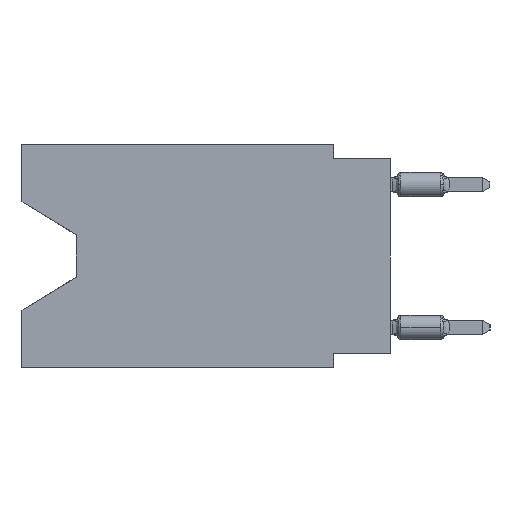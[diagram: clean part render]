
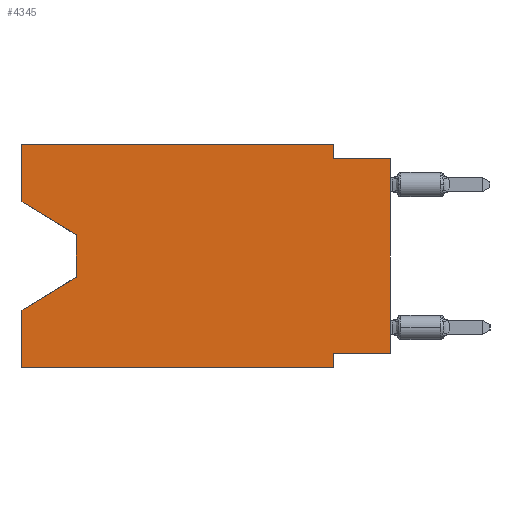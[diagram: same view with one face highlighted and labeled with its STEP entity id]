
A CAD part, left-side view. The second image highlights one B-rep face of the part: STEP entity #4345.
In plain terms, the highlighted planar face has unit normal (-1, 0, 0).
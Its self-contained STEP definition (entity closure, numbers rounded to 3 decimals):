
#278 = ORIENTED_EDGE ( 'NONE', *, *, #27530, .F. ) ;
#301 = LINE ( 'NONE', #47428, #45025 ) ;
#557 = PLANE ( 'NONE',  #7163 ) ;
#610 = DIRECTION ( 'NONE',  ( 0., -1., 0. ) ) ;
#781 = CARTESIAN_POINT ( 'NONE',  ( 0., 16.383, 0. ) ) ;
#833 = FACE_OUTER_BOUND ( 'NONE', #54676, .T. ) ;
#1397 = ORIENTED_EDGE ( 'NONE', *, *, #30987, .F. ) ;
#1782 = DIRECTION ( 'NONE',  ( 0., 0., -1. ) ) ;
#1792 = DIRECTION ( 'NONE',  ( 0., -1., 0. ) ) ;
#1962 = ORIENTED_EDGE ( 'NONE', *, *, #17357, .T. ) ;
#2312 = ORIENTED_EDGE ( 'NONE', *, *, #31524, .T. ) ;
#2405 = DIRECTION ( 'NONE',  ( 0., -1., 0. ) ) ;
#2544 = LINE ( 'NONE', #53923, #33160 ) ;
#3233 = CARTESIAN_POINT ( 'NONE',  ( 0., 2.54, -0.635 ) ) ;
#3855 = ORIENTED_EDGE ( 'NONE', *, *, #21883, .T. ) ;
#4100 = CARTESIAN_POINT ( 'NONE',  ( 0., 13.97, -5.893 ) ) ;
#4287 = LINE ( 'NONE', #25997, #41731 ) ;
#4345 = ADVANCED_FACE ( 'NONE', ( #833 ), #557, .F. ) ;
#5306 = ORIENTED_EDGE ( 'NONE', *, *, #22616, .T. ) ;
#5892 = VERTEX_POINT ( 'NONE', #55152 ) ;
#5977 = CARTESIAN_POINT ( 'NONE',  ( 0., 13.97, -4.013 ) ) ;
#6308 = LINE ( 'NONE', #40852, #37037 ) ;
#7163 = AXIS2_PLACEMENT_3D ( 'NONE', #44235, #23108, #9968 ) ;
#7332 = DIRECTION ( 'NONE',  ( 0., 0., -1. ) ) ;
#8209 = VERTEX_POINT ( 'NONE', #47959 ) ;
#9968 = DIRECTION ( 'NONE',  ( 0., 0., -1. ) ) ;
#11978 = DIRECTION ( 'NONE',  ( 0., -0.855, -0.519 ) ) ;
#12118 = EDGE_CURVE ( 'NONE', #30100, #5892, #39428, .T. ) ;
#13028 = LINE ( 'NONE', #52124, #28872 ) ;
#13922 = VECTOR ( 'NONE', #31520, 1000. ) ;
#14980 = CARTESIAN_POINT ( 'NONE',  ( 0., 0., -0.635 ) ) ;
#15195 = LINE ( 'NONE', #40882, #54041 ) ;
#15851 = EDGE_CURVE ( 'NONE', #8209, #45009, #21567, .T. ) ;
#16890 = DIRECTION ( 'NONE',  ( 0., 1., 0. ) ) ;
#16923 = EDGE_CURVE ( 'NONE', #54320, #50392, #301, .T. ) ;
#17357 = EDGE_CURVE ( 'NONE', #19999, #39767, #34508, .T. ) ;
#17637 = CARTESIAN_POINT ( 'NONE',  ( 0., 16.383, -2.546 ) ) ;
#18548 = VECTOR ( 'NONE', #610, 1000. ) ;
#18921 = CARTESIAN_POINT ( 'NONE',  ( 0., 0., -0.635 ) ) ;
#19999 = VERTEX_POINT ( 'NONE', #55900 ) ;
#20758 = VECTOR ( 'NONE', #2405, 1000. ) ;
#20968 = DIRECTION ( 'NONE',  ( 0., 0.855, -0.519 ) ) ;
#21567 = LINE ( 'NONE', #35801, #13922 ) ;
#21881 = VERTEX_POINT ( 'NONE', #14980 ) ;
#21883 = EDGE_CURVE ( 'NONE', #8209, #48928, #23825, .T. ) ;
#21969 = CARTESIAN_POINT ( 'NONE',  ( 0., 2.54, -9.271 ) ) ;
#22616 = EDGE_CURVE ( 'NONE', #54320, #21881, #4287, .T. ) ;
#23108 = DIRECTION ( 'NONE',  ( 1., 0., 0. ) ) ;
#23208 = LINE ( 'NONE', #18921, #23363 ) ;
#23363 = VECTOR ( 'NONE', #1792, 1000. ) ;
#23455 = DIRECTION ( 'NONE',  ( 0., 0., 1. ) ) ;
#23825 = LINE ( 'NONE', #44665, #20758 ) ;
#25997 = CARTESIAN_POINT ( 'NONE',  ( 0., 0., 0. ) ) ;
#27436 = ORIENTED_EDGE ( 'NONE', *, *, #28460, .F. ) ;
#27530 = EDGE_CURVE ( 'NONE', #50392, #48928, #15195, .T. ) ;
#28460 = EDGE_CURVE ( 'NONE', #5892, #51115, #2544, .T. ) ;
#28872 = VECTOR ( 'NONE', #7332, 1000. ) ;
#30100 = VERTEX_POINT ( 'NONE', #781 ) ;
#30987 = EDGE_CURVE ( 'NONE', #51115, #21881, #23208, .T. ) ;
#31520 = DIRECTION ( 'NONE',  ( 0., 0., 1. ) ) ;
#31524 = EDGE_CURVE ( 'NONE', #39767, #43185, #13028, .T. ) ;
#31718 = CARTESIAN_POINT ( 'NONE',  ( 0., 16.383, 0. ) ) ;
#33160 = VECTOR ( 'NONE', #50216, 1000. ) ;
#33634 = ORIENTED_EDGE ( 'NONE', *, *, #15851, .F. ) ;
#33817 = LINE ( 'NONE', #4100, #48170 ) ;
#34252 = CARTESIAN_POINT ( 'NONE',  ( 0., 0., -9.271 ) ) ;
#34508 = LINE ( 'NONE', #17637, #44068 ) ;
#35801 = CARTESIAN_POINT ( 'NONE',  ( 0., 16.383, 0. ) ) ;
#36679 = CARTESIAN_POINT ( 'NONE',  ( 0., 13.97, -5.893 ) ) ;
#37037 = VECTOR ( 'NONE', #23455, 1000. ) ;
#38468 = CARTESIAN_POINT ( 'NONE',  ( 0., 2.54, -9.906 ) ) ;
#39428 = LINE ( 'NONE', #31718, #18548 ) ;
#39670 = DIRECTION ( 'NONE',  ( 0., 0., 1. ) ) ;
#39767 = VERTEX_POINT ( 'NONE', #5977 ) ;
#40259 = ORIENTED_EDGE ( 'NONE', *, *, #50087, .F. ) ;
#40852 = CARTESIAN_POINT ( 'NONE',  ( 0., 16.383, 0. ) ) ;
#40882 = CARTESIAN_POINT ( 'NONE',  ( 0., 2.54, -9.906 ) ) ;
#41731 = VECTOR ( 'NONE', #39670, 1000. ) ;
#43185 = VERTEX_POINT ( 'NONE', #36679 ) ;
#44068 = VECTOR ( 'NONE', #11978, 1000. ) ;
#44235 = CARTESIAN_POINT ( 'NONE',  ( 0., 16.383, 0. ) ) ;
#44665 = CARTESIAN_POINT ( 'NONE',  ( 0., 16.383, -9.906 ) ) ;
#45009 = VERTEX_POINT ( 'NONE', #55305 ) ;
#45025 = VECTOR ( 'NONE', #16890, 1000. ) ;
#46824 = ORIENTED_EDGE ( 'NONE', *, *, #12118, .F. ) ;
#47428 = CARTESIAN_POINT ( 'NONE',  ( 0., 0., -9.271 ) ) ;
#47959 = CARTESIAN_POINT ( 'NONE',  ( 0., 16.383, -9.906 ) ) ;
#48170 = VECTOR ( 'NONE', #20968, 1000. ) ;
#48928 = VERTEX_POINT ( 'NONE', #38468 ) ;
#49050 = ORIENTED_EDGE ( 'NONE', *, *, #16923, .F. ) ;
#50087 = EDGE_CURVE ( 'NONE', #19999, #30100, #6308, .T. ) ;
#50216 = DIRECTION ( 'NONE',  ( 0., 0., -1. ) ) ;
#50392 = VERTEX_POINT ( 'NONE', #21969 ) ;
#51115 = VERTEX_POINT ( 'NONE', #3233 ) ;
#52124 = CARTESIAN_POINT ( 'NONE',  ( 0., 13.97, -4.013 ) ) ;
#52209 = EDGE_CURVE ( 'NONE', #43185, #45009, #33817, .T. ) ;
#53923 = CARTESIAN_POINT ( 'NONE',  ( 0., 2.54, 0. ) ) ;
#54041 = VECTOR ( 'NONE', #1782, 1000. ) ;
#54253 = ORIENTED_EDGE ( 'NONE', *, *, #52209, .T. ) ;
#54320 = VERTEX_POINT ( 'NONE', #34252 ) ;
#54676 = EDGE_LOOP ( 'NONE', ( #1962, #2312, #54253, #33634, #3855, #278, #49050, #5306, #1397, #27436, #46824, #40259 ) ) ;
#55152 = CARTESIAN_POINT ( 'NONE',  ( 0., 2.54, 0. ) ) ;
#55305 = CARTESIAN_POINT ( 'NONE',  ( 0., 16.383, -7.36 ) ) ;
#55900 = CARTESIAN_POINT ( 'NONE',  ( 0., 16.383, -2.546 ) ) ;
